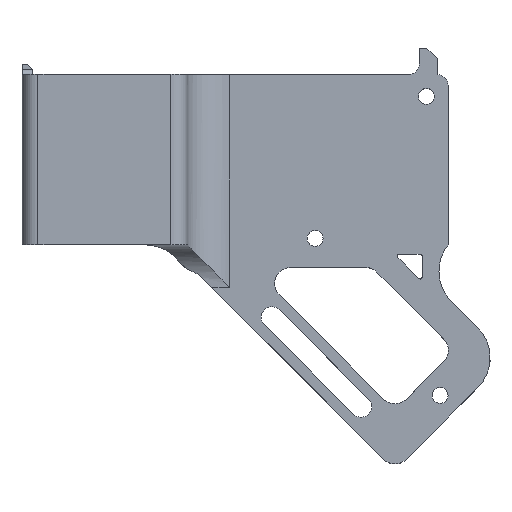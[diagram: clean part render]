
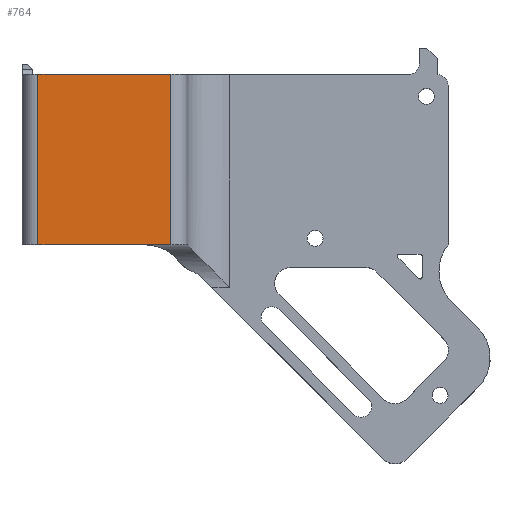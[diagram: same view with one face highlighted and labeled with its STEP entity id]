
A CAD part, top view. The second image highlights one B-rep face of the part: STEP entity #764.
In plain terms, the highlighted planar face has unit normal (0, 0, 1).
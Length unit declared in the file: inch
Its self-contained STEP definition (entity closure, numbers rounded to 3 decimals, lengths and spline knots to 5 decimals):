
#19 = EDGE_CURVE ( 'NONE', #2817, #899, #2104, .T. ) ;
#158 = PLANE ( 'NONE',  #654 ) ;
#171 = CARTESIAN_POINT ( 'NONE',  ( 0., 1.6, 1.75 ) ) ;
#174 = VECTOR ( 'NONE', #958, 39.37008 ) ;
#260 = CARTESIAN_POINT ( 'NONE',  ( 0.14436, 0., 1.75 ) ) ;
#337 = DIRECTION ( 'NONE',  ( 0., 1., 0. ) ) ;
#405 = CARTESIAN_POINT ( 'NONE',  ( 1.39436, 1.6, 1.75 ) ) ;
#654 = AXIS2_PLACEMENT_3D ( 'NONE', #2815, #975, #684 ) ;
#684 = DIRECTION ( 'NONE',  ( -1., 0., 0. ) ) ;
#691 = CARTESIAN_POINT ( 'NONE',  ( 0., 0., 1.75 ) ) ;
#750 = VECTOR ( 'NONE', #2835, 39.37008 ) ;
#764 = ADVANCED_FACE ( 'NONE', ( #2374 ), #158, .F. ) ;
#800 = EDGE_LOOP ( 'NONE', ( #2386, #2054, #1762, #2490 ) ) ;
#899 = VERTEX_POINT ( 'NONE', #2210 ) ;
#939 = VECTOR ( 'NONE', #2153, 39.37008 ) ;
#958 = DIRECTION ( 'NONE',  ( -1., 0., 0. ) ) ;
#975 = DIRECTION ( 'NONE',  ( 0., 0., -1. ) ) ;
#1269 = VECTOR ( 'NONE', #337, 39.37008 ) ;
#1544 = VERTEX_POINT ( 'NONE', #2457 ) ;
#1562 = EDGE_CURVE ( 'NONE', #3240, #2817, #1986, .T. ) ;
#1667 = LINE ( 'NONE', #260, #939 ) ;
#1762 = ORIENTED_EDGE ( 'NONE', *, *, #19, .T. ) ;
#1778 = CARTESIAN_POINT ( 'NONE',  ( 1.39436, 0., 1.75 ) ) ;
#1986 = LINE ( 'NONE', #2736, #1269 ) ;
#2054 = ORIENTED_EDGE ( 'NONE', *, *, #1562, .T. ) ;
#2104 = LINE ( 'NONE', #171, #174 ) ;
#2153 = DIRECTION ( 'NONE',  ( 0., -1., 0. ) ) ;
#2210 = CARTESIAN_POINT ( 'NONE',  ( 0.14436, 1.6, 1.75 ) ) ;
#2234 = EDGE_CURVE ( 'NONE', #899, #1544, #1667, .T. ) ;
#2274 = LINE ( 'NONE', #691, #750 ) ;
#2374 = FACE_OUTER_BOUND ( 'NONE', #800, .T. ) ;
#2386 = ORIENTED_EDGE ( 'NONE', *, *, #2980, .F. ) ;
#2457 = CARTESIAN_POINT ( 'NONE',  ( 0.14436, 0., 1.75 ) ) ;
#2490 = ORIENTED_EDGE ( 'NONE', *, *, #2234, .T. ) ;
#2736 = CARTESIAN_POINT ( 'NONE',  ( 1.39436, 0., 1.75 ) ) ;
#2815 = CARTESIAN_POINT ( 'NONE',  ( 0., 0., 1.75 ) ) ;
#2817 = VERTEX_POINT ( 'NONE', #405 ) ;
#2835 = DIRECTION ( 'NONE',  ( -1., 0., 0. ) ) ;
#2980 = EDGE_CURVE ( 'NONE', #3240, #1544, #2274, .T. ) ;
#3240 = VERTEX_POINT ( 'NONE', #1778 ) ;
